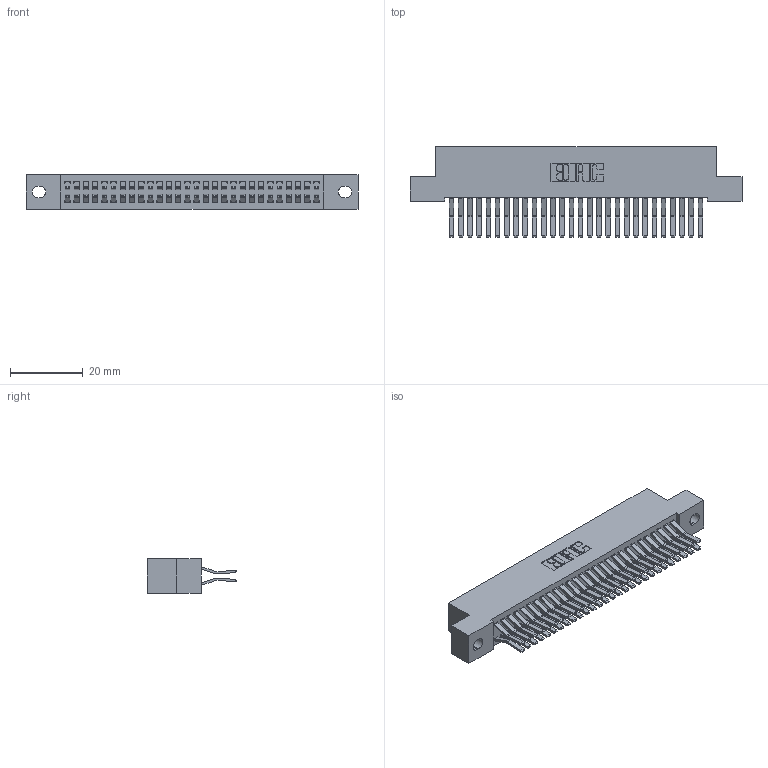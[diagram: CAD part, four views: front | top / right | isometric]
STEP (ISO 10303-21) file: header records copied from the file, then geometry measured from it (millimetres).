
FILE_DESCRIPTION (( 'STEP AP203' ), '1' );
FILE_NAME ('342-056-560-202.STEP', '2018-08-13T04:13:00', ( '' ), ( '' ), 'SwSTEP 2.0', 'SolidWorks 2016', '' );
FILE_SCHEMA (( 'CONFIG_CONTROL_DESIGN' ));
Length unit declared in the file: inch
Products named in the file (3): 342 Part_.128 Slot; 345-292-001_560 Tail; 342-056-560-202
Assembly tree (57 placements, depth 2):
  342-056-560-202
    342 Part_.128 Slot
    345-292-001_560 Tail  x56
Bounding box: 91.44 x 24.78 x 9.4 mm (x, y, z)
Volume: 8465.1 mm3; surface area: 14075.2 mm2
Topology: 57 solids, 57 shells, 3138 faces, 9327 edges, 6142 vertices
Faces by surface type: plane 2086, cylinder 1052
Entity records: 19915 total; most frequent: CARTESIAN_POINT 3318, ORIENTED_EDGE 3254, DIRECTION 2863, EDGE_CURVE 1627, LINE 1495, VECTOR 1495, VERTEX_POINT 1082, AXIS2_PLACEMENT_3D 684
